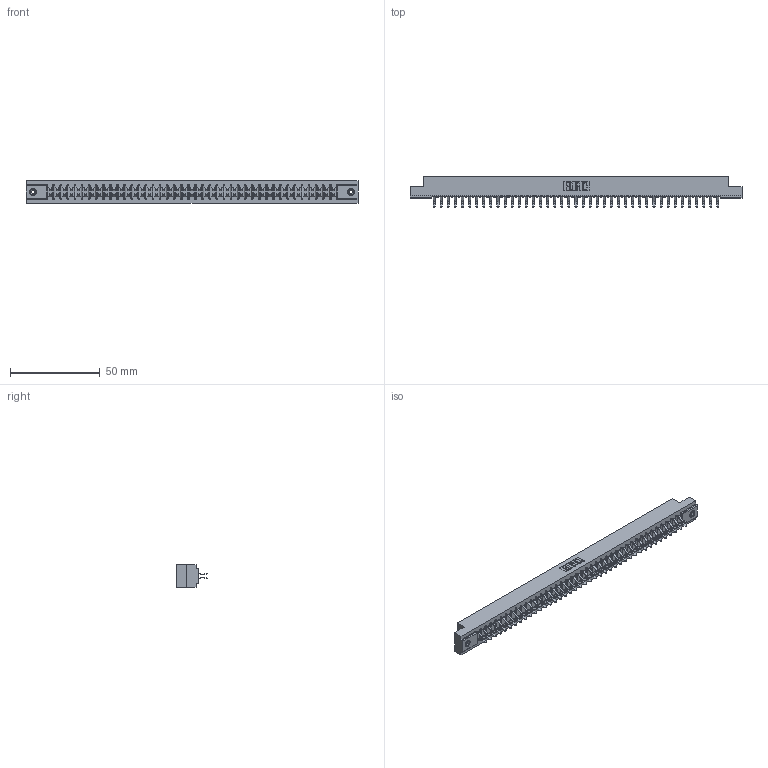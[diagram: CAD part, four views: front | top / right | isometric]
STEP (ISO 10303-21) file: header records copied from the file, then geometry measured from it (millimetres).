
FILE_DESCRIPTION (( 'STEP AP203' ), '1' );
FILE_NAME ('357-082-556-208.STEP', '2019-09-19T17:04:42', ( '' ), ( '' ), 'SwSTEP 2.0', 'SolidWorks 2016', '' );
FILE_SCHEMA (( 'CONFIG_CONTROL_DESIGN' ));
Length unit declared in the file: inch
Products named in the file (4): 307 Part_.156 Dia Mounting Holes; 307-290-001_556; 345-250-001_345-250-003-102; 357-082-556-208
Assembly tree (85 placements, depth 2):
  357-082-556-208
    307 Part_.156 Dia Mounting Holes
    307-290-001_556  x82
    345-250-001_345-250-003-102  x2
Bounding box: 185.47 x 16.97 x 12.7 mm (x, y, z)
Volume: 19694.2 mm3; surface area: 23881.3 mm2
Topology: 85 solids, 85 shells, 4320 faces, 12103 edges, 7838 vertices
Faces by surface type: plane 2808, cylinder 1412, sphere 84, cone 12, torus 4
Entity records: 37873 total; most frequent: CARTESIAN_POINT 6180, ORIENTED_EDGE 6118, DIRECTION 6063, EDGE_CURVE 3059, LINE 2345, VECTOR 2345, VERTEX_POINT 1976, AXIS2_PLACEMENT_3D 1859
